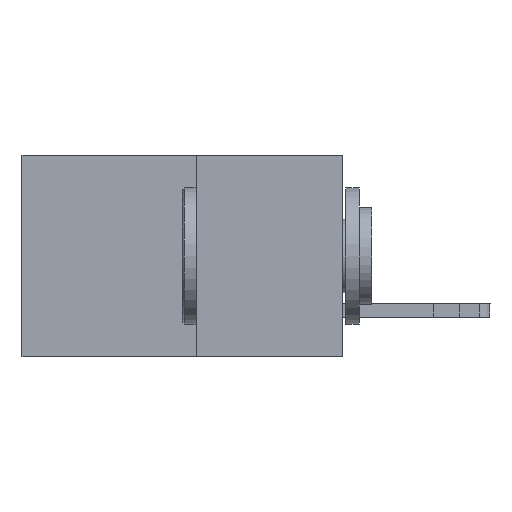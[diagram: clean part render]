
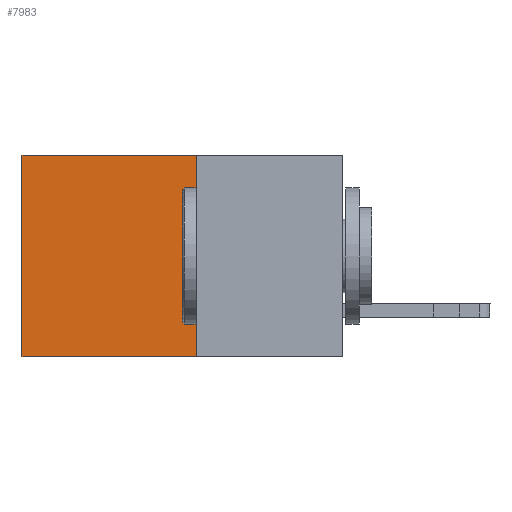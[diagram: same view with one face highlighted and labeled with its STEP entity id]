
A CAD part, left-side view. The second image highlights one B-rep face of the part: STEP entity #7983.
In plain terms, the highlighted planar face has unit normal (-1, 0, 0).
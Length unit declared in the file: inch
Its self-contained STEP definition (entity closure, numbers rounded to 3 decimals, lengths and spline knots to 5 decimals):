
#346 = CARTESIAN_POINT ( 'NONE',  ( 0.277, 0.59, 0. ) ) ;
#740 = DIRECTION ( 'NONE',  ( 0., 0., -1. ) ) ;
#1268 = DIRECTION ( 'NONE',  ( 0., 1., 0. ) ) ;
#1407 = ORIENTED_EDGE ( 'NONE', *, *, #3520, .F. ) ;
#1594 = CARTESIAN_POINT ( 'NONE',  ( 0.277, 0.27, -0.37 ) ) ;
#1630 = DIRECTION ( 'NONE',  ( 0., 1., 0. ) ) ;
#2252 = VERTEX_POINT ( 'NONE', #7659 ) ;
#2506 = FACE_OUTER_BOUND ( 'NONE', #11917, .T. ) ;
#2592 = VERTEX_POINT ( 'NONE', #6059 ) ;
#3323 = VECTOR ( 'NONE', #10969, 39.37008 ) ;
#3520 = EDGE_CURVE ( 'NONE', #2592, #2252, #12347, .T. ) ;
#3753 = VECTOR ( 'NONE', #1268, 39.37008 ) ;
#4468 = ORIENTED_EDGE ( 'NONE', *, *, #12329, .T. ) ;
#5016 = VERTEX_POINT ( 'NONE', #5832 ) ;
#5057 = LINE ( 'NONE', #10727, #8072 ) ;
#5670 = ORIENTED_EDGE ( 'NONE', *, *, #7670, .F. ) ;
#5832 = CARTESIAN_POINT ( 'NONE',  ( 0.277, 0.59, -0.37 ) ) ;
#6059 = CARTESIAN_POINT ( 'NONE',  ( 0.277, 0.27, 0. ) ) ;
#6340 = CARTESIAN_POINT ( 'NONE',  ( 0.277, 0.27, -0.37 ) ) ;
#7062 = VECTOR ( 'NONE', #740, 39.37008 ) ;
#7488 = DIRECTION ( 'NONE',  ( 0., 0., -1. ) ) ;
#7659 = CARTESIAN_POINT ( 'NONE',  ( 0.277, 0.27, -0.37 ) ) ;
#7670 = EDGE_CURVE ( 'NONE', #2252, #5016, #9452, .T. ) ;
#7983 = ADVANCED_FACE ( 'NONE', ( #2506 ), #13090, .F. ) ;
#8072 = VECTOR ( 'NONE', #1630, 39.37008 ) ;
#8085 = CARTESIAN_POINT ( 'NONE',  ( 0.277, 0.27, -0.37 ) ) ;
#8261 = AXIS2_PLACEMENT_3D ( 'NONE', #6340, #14184, #7488 ) ;
#9452 = LINE ( 'NONE', #8085, #3753 ) ;
#10642 = EDGE_CURVE ( 'NONE', #14103, #5016, #13052, .T. ) ;
#10727 = CARTESIAN_POINT ( 'NONE',  ( 0.277, 0.27, 0. ) ) ;
#10969 = DIRECTION ( 'NONE',  ( 0., 0., -1. ) ) ;
#10970 = CARTESIAN_POINT ( 'NONE',  ( 0.277, 0.59, -0.37 ) ) ;
#11001 = ORIENTED_EDGE ( 'NONE', *, *, #10642, .T. ) ;
#11917 = EDGE_LOOP ( 'NONE', ( #11001, #5670, #1407, #4468 ) ) ;
#12329 = EDGE_CURVE ( 'NONE', #2592, #14103, #5057, .T. ) ;
#12347 = LINE ( 'NONE', #1594, #3323 ) ;
#13052 = LINE ( 'NONE', #10970, #7062 ) ;
#13090 = PLANE ( 'NONE',  #8261 ) ;
#14103 = VERTEX_POINT ( 'NONE', #346 ) ;
#14184 = DIRECTION ( 'NONE',  ( 1., 0., 0. ) ) ;
